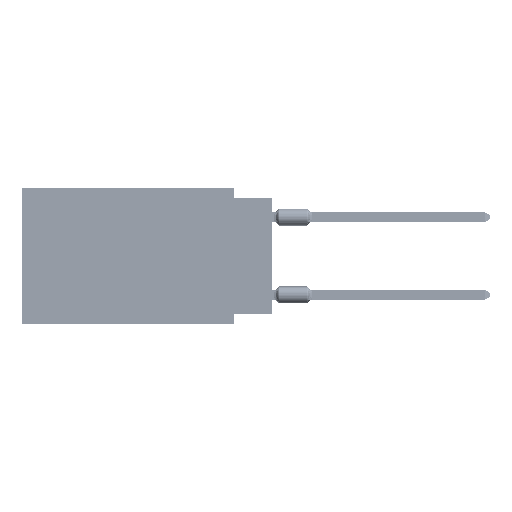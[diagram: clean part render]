
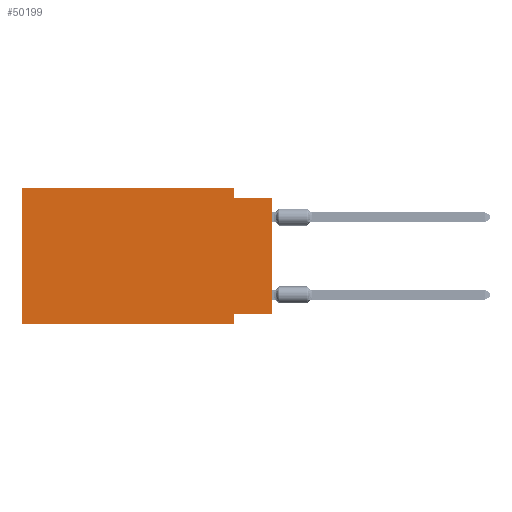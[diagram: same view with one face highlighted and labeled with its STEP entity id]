
A CAD part, left-side view. The second image highlights one B-rep face of the part: STEP entity #50199.
In plain terms, the highlighted planar face has unit normal (-1, 0, 0).
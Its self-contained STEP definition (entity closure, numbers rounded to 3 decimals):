
#608 = CARTESIAN_POINT ( 'NONE',  ( 0., 2.54, -0.635 ) ) ;
#851 = CARTESIAN_POINT ( 'NONE',  ( 0., 0., -8.255 ) ) ;
#2817 = VECTOR ( 'NONE', #111531, 1000. ) ;
#4982 = CARTESIAN_POINT ( 'NONE',  ( 0., 16.383, 0. ) ) ;
#6166 = AXIS2_PLACEMENT_3D ( 'NONE', #56871, #73371, #11394 ) ;
#6292 = LINE ( 'NONE', #14843, #2817 ) ;
#8168 = DIRECTION ( 'NONE',  ( 0., 0., -1. ) ) ;
#9212 = VECTOR ( 'NONE', #107552, 1000. ) ;
#10131 = CARTESIAN_POINT ( 'NONE',  ( 0., 16.383, -8.89 ) ) ;
#10364 = VECTOR ( 'NONE', #86350, 1000. ) ;
#11394 = DIRECTION ( 'NONE',  ( 0., 0., -1. ) ) ;
#12045 = EDGE_CURVE ( 'NONE', #59924, #35647, #13359, .T. ) ;
#13359 = LINE ( 'NONE', #82725, #44205 ) ;
#14843 = CARTESIAN_POINT ( 'NONE',  ( 0., 16.383, 0. ) ) ;
#17826 = EDGE_CURVE ( 'NONE', #59924, #68366, #105738, .T. ) ;
#23520 = VERTEX_POINT ( 'NONE', #608 ) ;
#25660 = CARTESIAN_POINT ( 'NONE',  ( 0., 0., -0.635 ) ) ;
#25723 = VERTEX_POINT ( 'NONE', #70314 ) ;
#28027 = CARTESIAN_POINT ( 'NONE',  ( 0., 2.54, -8.255 ) ) ;
#29487 = CARTESIAN_POINT ( 'NONE',  ( 0., 0., 0. ) ) ;
#30204 = DIRECTION ( 'NONE',  ( 0., 0., -1. ) ) ;
#30382 = VECTOR ( 'NONE', #52804, 1000. ) ;
#30706 = FACE_OUTER_BOUND ( 'NONE', #101106, .T. ) ;
#31311 = EDGE_CURVE ( 'NONE', #81521, #55393, #6292, .T. ) ;
#32993 = EDGE_CURVE ( 'NONE', #81521, #25723, #104004, .T. ) ;
#35647 = VERTEX_POINT ( 'NONE', #28027 ) ;
#37614 = CARTESIAN_POINT ( 'NONE',  ( 0., 2.54, 0. ) ) ;
#38083 = VECTOR ( 'NONE', #30204, 1000. ) ;
#38428 = ORIENTED_EDGE ( 'NONE', *, *, #46938, .F. ) ;
#39270 = CARTESIAN_POINT ( 'NONE',  ( 0., 16.383, 0. ) ) ;
#40521 = VECTOR ( 'NONE', #8168, 1000. ) ;
#44205 = VECTOR ( 'NONE', #91832, 1000. ) ;
#44358 = ORIENTED_EDGE ( 'NONE', *, *, #32993, .T. ) ;
#46938 = EDGE_CURVE ( 'NONE', #93072, #23520, #80815, .T. ) ;
#50199 = ADVANCED_FACE ( 'NONE', ( #30706 ), #83008, .F. ) ;
#50761 = EDGE_CURVE ( 'NONE', #35647, #25723, #83280, .T. ) ;
#52243 = CARTESIAN_POINT ( 'NONE',  ( 0., 0., -0.635 ) ) ;
#52804 = DIRECTION ( 'NONE',  ( 0., -1., 0. ) ) ;
#54522 = DIRECTION ( 'NONE',  ( 0., 0., 1. ) ) ;
#55393 = VERTEX_POINT ( 'NONE', #4982 ) ;
#56871 = CARTESIAN_POINT ( 'NONE',  ( 0., 16.383, 0. ) ) ;
#59924 = VERTEX_POINT ( 'NONE', #851 ) ;
#60495 = CARTESIAN_POINT ( 'NONE',  ( 0., 2.54, -8.89 ) ) ;
#61955 = ORIENTED_EDGE ( 'NONE', *, *, #12045, .F. ) ;
#62643 = CARTESIAN_POINT ( 'NONE',  ( 0., 2.54, 0. ) ) ;
#63931 = VECTOR ( 'NONE', #54522, 1000. ) ;
#68186 = LINE ( 'NONE', #52243, #30382 ) ;
#68366 = VERTEX_POINT ( 'NONE', #25660 ) ;
#70314 = CARTESIAN_POINT ( 'NONE',  ( 0., 2.54, -8.89 ) ) ;
#73371 = DIRECTION ( 'NONE',  ( 1., 0., 0. ) ) ;
#74528 = ORIENTED_EDGE ( 'NONE', *, *, #82501, .F. ) ;
#78453 = ORIENTED_EDGE ( 'NONE', *, *, #50761, .F. ) ;
#80455 = ORIENTED_EDGE ( 'NONE', *, *, #101773, .F. ) ;
#80815 = LINE ( 'NONE', #37614, #38083 ) ;
#81521 = VERTEX_POINT ( 'NONE', #102894 ) ;
#82480 = LINE ( 'NONE', #39270, #9212 ) ;
#82501 = EDGE_CURVE ( 'NONE', #55393, #93072, #82480, .T. ) ;
#82725 = CARTESIAN_POINT ( 'NONE',  ( 0., 0., -8.255 ) ) ;
#83008 = PLANE ( 'NONE',  #6166 ) ;
#83280 = LINE ( 'NONE', #60495, #40521 ) ;
#84378 = ORIENTED_EDGE ( 'NONE', *, *, #31311, .F. ) ;
#86350 = DIRECTION ( 'NONE',  ( 0., -1., 0. ) ) ;
#91832 = DIRECTION ( 'NONE',  ( 0., 1., 0. ) ) ;
#93072 = VERTEX_POINT ( 'NONE', #62643 ) ;
#101106 = EDGE_LOOP ( 'NONE', ( #105745, #80455, #38428, #74528, #84378, #44358, #78453, #61955 ) ) ;
#101773 = EDGE_CURVE ( 'NONE', #23520, #68366, #68186, .T. ) ;
#102894 = CARTESIAN_POINT ( 'NONE',  ( 0., 16.383, -8.89 ) ) ;
#104004 = LINE ( 'NONE', #10131, #10364 ) ;
#105738 = LINE ( 'NONE', #29487, #63931 ) ;
#105745 = ORIENTED_EDGE ( 'NONE', *, *, #17826, .T. ) ;
#107552 = DIRECTION ( 'NONE',  ( 0., -1., 0. ) ) ;
#111531 = DIRECTION ( 'NONE',  ( 0., 0., 1. ) ) ;
